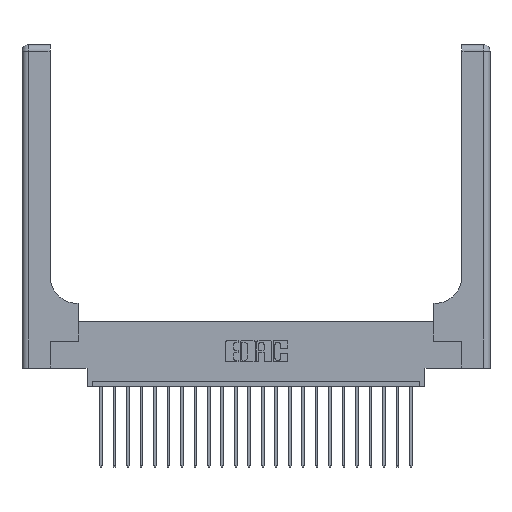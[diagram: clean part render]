
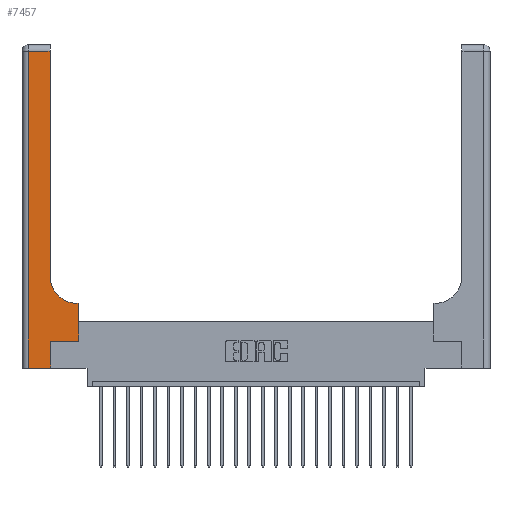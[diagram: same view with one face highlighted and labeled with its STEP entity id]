
A CAD part, top view. The second image highlights one B-rep face of the part: STEP entity #7457.
In plain terms, the highlighted planar face has unit normal (0, 0, 1).
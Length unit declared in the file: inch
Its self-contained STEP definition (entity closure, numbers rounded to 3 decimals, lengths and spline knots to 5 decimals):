
#102 = EDGE_CURVE ( 'NONE', #9423, #4968, #17785, .T. ) ;
#471 = LINE ( 'NONE', #1761, #18267 ) ;
#916 = LINE ( 'NONE', #16214, #1465 ) ;
#1247 = ORIENTED_EDGE ( 'NONE', *, *, #14868, .T. ) ;
#1365 = DIRECTION ( 'NONE',  ( 0., 0., -1. ) ) ;
#1465 = VECTOR ( 'NONE', #2350, 39.37008 ) ;
#1480 = LINE ( 'NONE', #18812, #6426 ) ;
#1761 = CARTESIAN_POINT ( 'NONE',  ( 0.265, 0., 0.37 ) ) ;
#2231 = CARTESIAN_POINT ( 'NONE',  ( 0.06, 0., 0.37 ) ) ;
#2255 = DIRECTION ( 'NONE',  ( 1., 0., 0. ) ) ;
#2350 = DIRECTION ( 'NONE',  ( 1., 0., 0. ) ) ;
#2622 = ORIENTED_EDGE ( 'NONE', *, *, #3267, .T. ) ;
#2706 = ORIENTED_EDGE ( 'NONE', *, *, #9515, .T. ) ;
#2992 = VERTEX_POINT ( 'NONE', #20092 ) ;
#3108 = DIRECTION ( 'NONE',  ( 1., 0., 0. ) ) ;
#3267 = EDGE_CURVE ( 'NONE', #12101, #2992, #22325, .T. ) ;
#3336 = CARTESIAN_POINT ( 'NONE',  ( 0.51, 0.6, 0.37 ) ) ;
#4213 = CARTESIAN_POINT ( 'NONE',  ( 0.265, 0., 0.37 ) ) ;
#4968 = VERTEX_POINT ( 'NONE', #4213 ) ;
#5367 = DIRECTION ( 'NONE',  ( -1., 0., 0. ) ) ;
#5740 = VECTOR ( 'NONE', #5367, 39.37008 ) ;
#6135 = VERTEX_POINT ( 'NONE', #21644 ) ;
#6317 = VERTEX_POINT ( 'NONE', #18958 ) ;
#6426 = VECTOR ( 'NONE', #13621, 39.37008 ) ;
#6781 = AXIS2_PLACEMENT_3D ( 'NONE', #11894, #1365, #3108 ) ;
#7205 = CARTESIAN_POINT ( 'NONE',  ( 0.26, 0.6, 0.37 ) ) ;
#7228 = ORIENTED_EDGE ( 'NONE', *, *, #17232, .T. ) ;
#7457 = ADVANCED_FACE ( 'NONE', ( #15732 ), #7595, .F. ) ;
#7489 = ORIENTED_EDGE ( 'NONE', *, *, #20148, .T. ) ;
#7595 = PLANE ( 'NONE',  #9414 ) ;
#7989 = LINE ( 'NONE', #14788, #17581 ) ;
#8121 = CARTESIAN_POINT ( 'NONE',  ( 0.265, 0.25, 0.37 ) ) ;
#9369 = DIRECTION ( 'NONE',  ( 0., 0., -1. ) ) ;
#9414 = AXIS2_PLACEMENT_3D ( 'NONE', #19815, #9369, #21596 ) ;
#9423 = VERTEX_POINT ( 'NONE', #2231 ) ;
#9515 = EDGE_CURVE ( 'NONE', #2992, #6317, #7989, .T. ) ;
#9710 = CARTESIAN_POINT ( 'NONE',  ( 0.528, 0.25, 0.37 ) ) ;
#10215 = LINE ( 'NONE', #22426, #22505 ) ;
#10471 = CARTESIAN_POINT ( 'NONE',  ( 0.528, 0.25, 0.37 ) ) ;
#11225 = VERTEX_POINT ( 'NONE', #15182 ) ;
#11263 = VECTOR ( 'NONE', #15135, 39.37008 ) ;
#11894 = CARTESIAN_POINT ( 'NONE',  ( 0.51, 0.85, 0.37 ) ) ;
#12101 = VERTEX_POINT ( 'NONE', #3336 ) ;
#12388 = VECTOR ( 'NONE', #2255, 39.37008 ) ;
#13177 = EDGE_CURVE ( 'NONE', #6135, #9423, #10215, .T. ) ;
#13621 = DIRECTION ( 'NONE',  ( -1., 0., 0. ) ) ;
#14235 = DIRECTION ( 'NONE',  ( 0., 1., 0. ) ) ;
#14788 = CARTESIAN_POINT ( 'NONE',  ( 0.26, 3., 0.37 ) ) ;
#14868 = EDGE_CURVE ( 'NONE', #11225, #12101, #18317, .T. ) ;
#15135 = DIRECTION ( 'NONE',  ( 0., 1., 0. ) ) ;
#15182 = CARTESIAN_POINT ( 'NONE',  ( 0.528, 0.6, 0.37 ) ) ;
#15732 = FACE_OUTER_BOUND ( 'NONE', #20055, .T. ) ;
#16214 = CARTESIAN_POINT ( 'NONE',  ( 0.265, 0.25, 0.37 ) ) ;
#16469 = DIRECTION ( 'NONE',  ( 0., 1., 0. ) ) ;
#16691 = ORIENTED_EDGE ( 'NONE', *, *, #102, .T. ) ;
#17232 = EDGE_CURVE ( 'NONE', #4968, #17406, #471, .T. ) ;
#17406 = VERTEX_POINT ( 'NONE', #8121 ) ;
#17581 = VECTOR ( 'NONE', #16469, 39.37008 ) ;
#17785 = LINE ( 'NONE', #20864, #12388 ) ;
#18267 = VECTOR ( 'NONE', #14235, 39.37008 ) ;
#18317 = LINE ( 'NONE', #7205, #5740 ) ;
#18812 = CARTESIAN_POINT ( 'NONE',  ( 0., 2.94, 0.37 ) ) ;
#18958 = CARTESIAN_POINT ( 'NONE',  ( 0.26, 2.94, 0.37 ) ) ;
#18984 = DIRECTION ( 'NONE',  ( 0., -1., 0. ) ) ;
#19144 = EDGE_CURVE ( 'NONE', #6317, #6135, #1480, .T. ) ;
#19815 = CARTESIAN_POINT ( 'NONE',  ( 0., 3., 0.37 ) ) ;
#20055 = EDGE_LOOP ( 'NONE', ( #2706, #20677, #21363, #16691, #7228, #7489, #21831, #1247, #2622 ) ) ;
#20092 = CARTESIAN_POINT ( 'NONE',  ( 0.26, 0.85, 0.37 ) ) ;
#20148 = EDGE_CURVE ( 'NONE', #17406, #20766, #916, .T. ) ;
#20529 = LINE ( 'NONE', #9710, #11263 ) ;
#20677 = ORIENTED_EDGE ( 'NONE', *, *, #19144, .T. ) ;
#20766 = VERTEX_POINT ( 'NONE', #10471 ) ;
#20864 = CARTESIAN_POINT ( 'NONE',  ( 0., 0., 0.37 ) ) ;
#21363 = ORIENTED_EDGE ( 'NONE', *, *, #13177, .T. ) ;
#21596 = DIRECTION ( 'NONE',  ( -1., 0., 0. ) ) ;
#21644 = CARTESIAN_POINT ( 'NONE',  ( 0.06, 2.94, 0.37 ) ) ;
#21831 = ORIENTED_EDGE ( 'NONE', *, *, #22038, .T. ) ;
#22038 = EDGE_CURVE ( 'NONE', #20766, #11225, #20529, .T. ) ;
#22325 = CIRCLE ( 'NONE', #6781, 0.25 ) ;
#22426 = CARTESIAN_POINT ( 'NONE',  ( 0.06, 3., 0.37 ) ) ;
#22505 = VECTOR ( 'NONE', #18984, 39.37008 ) ;
